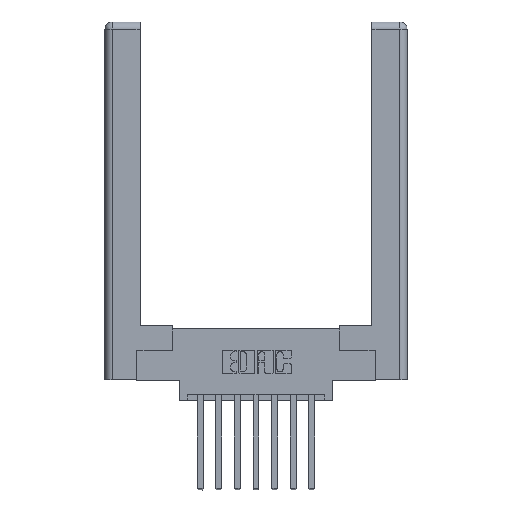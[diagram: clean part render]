
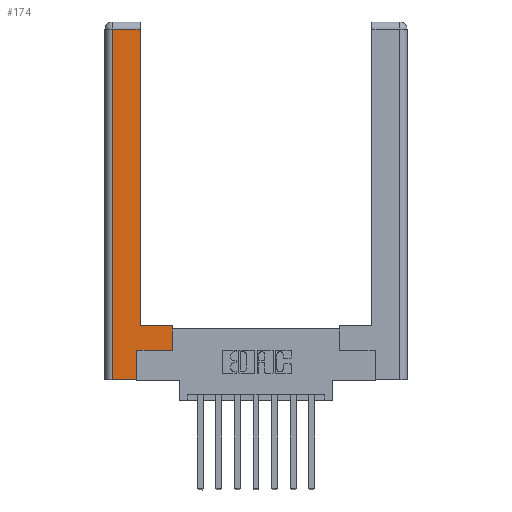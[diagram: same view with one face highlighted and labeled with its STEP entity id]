
A CAD part, top view. The second image highlights one B-rep face of the part: STEP entity #174.
In plain terms, the highlighted planar face has unit normal (0, 0, 1).
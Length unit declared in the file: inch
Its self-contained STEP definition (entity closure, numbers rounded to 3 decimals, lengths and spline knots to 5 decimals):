
#127 = AXIS2_PLACEMENT_3D ( 'NONE', #2680, #3735, #9458 ) ;
#174 = ADVANCED_FACE ( 'NONE', ( #4623 ), #7488, .F. ) ;
#197 = ORIENTED_EDGE ( 'NONE', *, *, #11810, .T. ) ;
#440 = LINE ( 'NONE', #6179, #2418 ) ;
#623 = ORIENTED_EDGE ( 'NONE', *, *, #6875, .T. ) ;
#626 = VERTEX_POINT ( 'NONE', #5577 ) ;
#696 = VECTOR ( 'NONE', #10829, 39.37008 ) ;
#994 = VECTOR ( 'NONE', #11406, 39.37008 ) ;
#1182 = VERTEX_POINT ( 'NONE', #3833 ) ;
#1224 = EDGE_LOOP ( 'NONE', ( #10243, #9964, #10207, #197, #623, #5811, #7183, #2086 ) ) ;
#1543 = DIRECTION ( 'NONE',  ( 1., 0., 0. ) ) ;
#1809 = CARTESIAN_POINT ( 'NONE',  ( 0.265, 0., 0. ) ) ;
#1858 = LINE ( 'NONE', #4369, #9289 ) ;
#2086 = ORIENTED_EDGE ( 'NONE', *, *, #3659, .T. ) ;
#2418 = VECTOR ( 'NONE', #9852, 39.37008 ) ;
#2420 = VECTOR ( 'NONE', #5162, 39.37008 ) ;
#2568 = VECTOR ( 'NONE', #1543, 39.37008 ) ;
#2680 = CARTESIAN_POINT ( 'NONE',  ( 0., 0., 0. ) ) ;
#2915 = EDGE_CURVE ( 'NONE', #8576, #10859, #8416, .T. ) ;
#2971 = LINE ( 'NONE', #5559, #994 ) ;
#3049 = CARTESIAN_POINT ( 'NONE',  ( 0.565, 0.245, 0. ) ) ;
#3267 = DIRECTION ( 'NONE',  ( 0., 1., 0. ) ) ;
#3659 = EDGE_CURVE ( 'NONE', #5620, #626, #2971, .T. ) ;
#3735 = DIRECTION ( 'NONE',  ( 0., 0., -1. ) ) ;
#3807 = CARTESIAN_POINT ( 'NONE',  ( 0.565, 0.45, 0. ) ) ;
#3833 = CARTESIAN_POINT ( 'NONE',  ( 0.0615, 2.94, 0. ) ) ;
#4369 = CARTESIAN_POINT ( 'NONE',  ( 0.0615, 0., 0. ) ) ;
#4502 = CARTESIAN_POINT ( 'NONE',  ( 0.0615, 0., 0. ) ) ;
#4623 = FACE_OUTER_BOUND ( 'NONE', #1224, .T. ) ;
#4915 = EDGE_CURVE ( 'NONE', #1182, #5534, #1858, .T. ) ;
#5157 = LINE ( 'NONE', #7250, #2568 ) ;
#5162 = DIRECTION ( 'NONE',  ( -1., 0., 0. ) ) ;
#5309 = CARTESIAN_POINT ( 'NONE',  ( 0.295, 3., 0. ) ) ;
#5451 = EDGE_CURVE ( 'NONE', #626, #6235, #9274, .T. ) ;
#5534 = VERTEX_POINT ( 'NONE', #4502 ) ;
#5559 = CARTESIAN_POINT ( 'NONE',  ( 0.295, 0.45, 0. ) ) ;
#5577 = CARTESIAN_POINT ( 'NONE',  ( 0.295, 0.45, 0. ) ) ;
#5620 = VERTEX_POINT ( 'NONE', #3807 ) ;
#5811 = ORIENTED_EDGE ( 'NONE', *, *, #2915, .T. ) ;
#6179 = CARTESIAN_POINT ( 'NONE',  ( 0.265, 0.245, 0. ) ) ;
#6235 = VERTEX_POINT ( 'NONE', #7187 ) ;
#6442 = CARTESIAN_POINT ( 'NONE',  ( 0.565, 0.45, 0. ) ) ;
#6875 = EDGE_CURVE ( 'NONE', #12289, #8576, #440, .T. ) ;
#7183 = ORIENTED_EDGE ( 'NONE', *, *, #7702, .T. ) ;
#7187 = CARTESIAN_POINT ( 'NONE',  ( 0.295, 2.94, 0. ) ) ;
#7250 = CARTESIAN_POINT ( 'NONE',  ( 0.265, 0., 0. ) ) ;
#7488 = PLANE ( 'NONE',  #127 ) ;
#7702 = EDGE_CURVE ( 'NONE', #10859, #5620, #7942, .T. ) ;
#7942 = LINE ( 'NONE', #6442, #11157 ) ;
#8159 = DIRECTION ( 'NONE',  ( 0., -1., 0. ) ) ;
#8416 = LINE ( 'NONE', #3049, #696 ) ;
#8576 = VERTEX_POINT ( 'NONE', #9080 ) ;
#8656 = VECTOR ( 'NONE', #3267, 39.37008 ) ;
#9080 = CARTESIAN_POINT ( 'NONE',  ( 0.265, 0.245, 0. ) ) ;
#9274 = LINE ( 'NONE', #5309, #8656 ) ;
#9289 = VECTOR ( 'NONE', #8159, 39.37008 ) ;
#9458 = DIRECTION ( 'NONE',  ( -1., 0., 0. ) ) ;
#9834 = CARTESIAN_POINT ( 'NONE',  ( 0.565, 0.245, 0. ) ) ;
#9852 = DIRECTION ( 'NONE',  ( 0., 1., 0. ) ) ;
#9964 = ORIENTED_EDGE ( 'NONE', *, *, #11755, .T. ) ;
#10063 = CARTESIAN_POINT ( 'NONE',  ( 0.0615, 2.94, 0. ) ) ;
#10207 = ORIENTED_EDGE ( 'NONE', *, *, #4915, .T. ) ;
#10243 = ORIENTED_EDGE ( 'NONE', *, *, #5451, .T. ) ;
#10829 = DIRECTION ( 'NONE',  ( 1., 0., 0. ) ) ;
#10859 = VERTEX_POINT ( 'NONE', #9834 ) ;
#11157 = VECTOR ( 'NONE', #11192, 39.37008 ) ;
#11192 = DIRECTION ( 'NONE',  ( 0., 1., 0. ) ) ;
#11406 = DIRECTION ( 'NONE',  ( -1., 0., 0. ) ) ;
#11755 = EDGE_CURVE ( 'NONE', #6235, #1182, #12144, .T. ) ;
#11810 = EDGE_CURVE ( 'NONE', #5534, #12289, #5157, .T. ) ;
#12144 = LINE ( 'NONE', #10063, #2420 ) ;
#12289 = VERTEX_POINT ( 'NONE', #1809 ) ;
